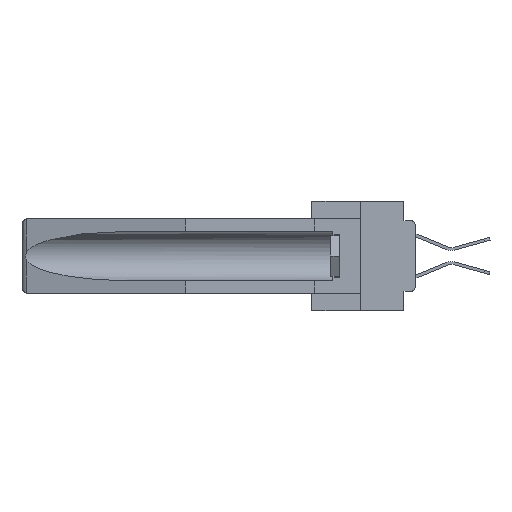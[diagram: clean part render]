
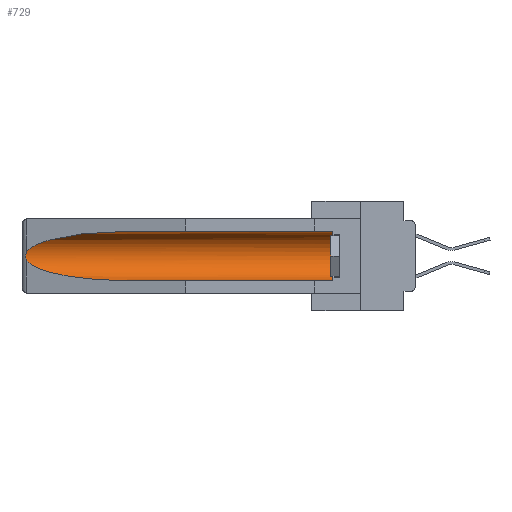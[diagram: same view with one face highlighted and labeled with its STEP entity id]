
A CAD part, left-side view. The second image highlights one B-rep face of the part: STEP entity #729.
In plain terms, the highlighted cylindrical face has radius 2.857 mm (diameter 5.715 mm), a partial arc.
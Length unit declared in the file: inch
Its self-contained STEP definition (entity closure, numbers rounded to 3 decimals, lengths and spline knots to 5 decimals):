
#336 = CARTESIAN_POINT ( 'NONE',  ( 0.155, -0.30754, -0.284 ) ) ;
#729 = ADVANCED_FACE ( 'NONE', ( #14350 ), #22308, .F. ) ;
#968 = CARTESIAN_POINT ( 'NONE',  ( 0.155, 1.07973, -0.284 ) ) ;
#1358 = ORIENTED_EDGE ( 'NONE', *, *, #25346, .T. ) ;
#1753 = EDGE_CURVE ( 'NONE', #28418, #22127, #26132, .T. ) ;
#1892 = DIRECTION ( 'NONE',  ( 0., 1., 0. ) ) ;
#1933 = CARTESIAN_POINT ( 'NONE',  ( 0.26654, 1.53092, -0.15636 ) ) ;
#2085 = CARTESIAN_POINT ( 'NONE',  ( 0.2675, 1.53308, -0.16763 ) ) ;
#2621 = CARTESIAN_POINT ( 'NONE',  ( 0.25451, 1.48313, -0.24835 ) ) ;
#4347 = CARTESIAN_POINT ( 'NONE',  ( 0.155, -0.30754, -0.1715 ) ) ;
#4593 = VECTOR ( 'NONE', #5719, 39.37008 ) ;
#5233 = CARTESIAN_POINT ( 'NONE',  ( 0.155, 1.07973, -0.284 ) ) ;
#5643 = CARTESIAN_POINT ( 'NONE',  ( 0.155, -0.30754, -0.059 ) ) ;
#5719 = DIRECTION ( 'NONE',  ( 0., 1., 0. ) ) ;
#6481 = ORIENTED_EDGE ( 'NONE', *, *, #31178, .T. ) ;
#7720 = EDGE_LOOP ( 'NONE', ( #1358, #6481, #26420, #23361, #24828, #29363 ) ) ;
#8289 = VERTEX_POINT ( 'NONE', #15054 ) ;
#8754 = LINE ( 'NONE', #5643, #9029 ) ;
#9025 = VERTEX_POINT ( 'NONE', #968 ) ;
#9029 = VECTOR ( 'NONE', #1892, 39.37008 ) ;
#10330 = CARTESIAN_POINT ( 'NONE',  ( 0.21114, 1.30732, -0.284 ) ) ;
#11923 = CARTESIAN_POINT ( 'NONE',  ( 0.26537, 1.52718, -0.19328 ) ) ;
#12438 = CARTESIAN_POINT ( 'NONE',  ( 0.155, 0.126, -0.1715 ) ) ;
#13761 = B_SPLINE_CURVE_WITH_KNOTS ( 'NONE', 3,
 ( #20060, #27481, #1933, #21863, #2085, #14536, #29668, #31794, #24609, #11923 ),
 .UNSPECIFIED., .F., .F.,
 ( 4, 2, 2, 2, 4 ),
 ( 0., 0.00029, 0.00058, 0.00087, 0.00117 ),
 .UNSPECIFIED. ) ;
#14350 = FACE_OUTER_BOUND ( 'NONE', #7720, .T. ) ;
#14536 = CARTESIAN_POINT ( 'NONE',  ( 0.2675, 1.53308, -0.17534 ) ) ;
#15054 = CARTESIAN_POINT ( 'NONE',  ( 0.26537, 1.52718, -0.14972 ) ) ;
#15680 = CARTESIAN_POINT ( 'NONE',  ( 0.26537, 1.52718, -0.19328 ) ) ;
#17288 = AXIS2_PLACEMENT_3D ( 'NONE', #12438, #24976, #30194 ) ;
#19222 = CARTESIAN_POINT ( 'NONE',  ( 0.155, 0.126, -0.284 ) ) ;
#19364 = CARTESIAN_POINT ( 'NONE',  ( 0.21114, 1.30732, -0.059 ) ) ;
#19534 = CARTESIAN_POINT ( 'NONE',  ( 0.26537, 1.52718, -0.14972 ) ) ;
#20060 = CARTESIAN_POINT ( 'NONE',  ( 0.26537, 1.52718, -0.14972 ) ) ;
#20889 = EDGE_CURVE ( 'NONE', #28418, #9025, #22883, .T. ) ;
#21863 = CARTESIAN_POINT ( 'NONE',  ( 0.2673, 1.5327, -0.16383 ) ) ;
#22005 = DIRECTION ( 'NONE',  ( 0., 0., 1. ) ) ;
#22127 = VERTEX_POINT ( 'NONE', #32031 ) ;
#22308 = CYLINDRICAL_SURFACE ( 'NONE', #28158, 0.1125 ) ;
#22883 = LINE ( 'NONE', #336, #4593 ) ;
#23361 = ORIENTED_EDGE ( 'NONE', *, *, #20889, .F. ) ;
#23392 = VERTEX_POINT ( 'NONE', #27031 ) ;
#24244 = CARTESIAN_POINT ( 'NONE',  ( 0.155, 1.07973, -0.059 ) ) ;
#24609 = CARTESIAN_POINT ( 'NONE',  ( 0.26597, 1.5296, -0.19026 ) ) ;
#24828 = ORIENTED_EDGE ( 'NONE', *, *, #1753, .T. ) ;
#24976 = DIRECTION ( 'NONE',  ( 0., -1., 0. ) ) ;
#25177 =( BOUNDED_CURVE ( )  B_SPLINE_CURVE ( 3, ( #24244, #19364, #27319, #19534 ),
 .UNSPECIFIED., .F., .T. ) 
 B_SPLINE_CURVE_WITH_KNOTS ( ( 4, 4 ),
 ( 4.71239, 6.08839 ),
 .UNSPECIFIED. ) 
 CURVE ( )  GEOMETRIC_REPRESENTATION_ITEM ( )  RATIONAL_B_SPLINE_CURVE ( ( 1., 0.848, 0.848, 1. ) ) 
 REPRESENTATION_ITEM ( '' )  );
#25346 = EDGE_CURVE ( 'NONE', #23392, #8289, #25177, .T. ) ;
#25470 = CARTESIAN_POINT ( 'NONE',  ( 0.26537, 1.52718, -0.19328 ) ) ;
#25883 = EDGE_CURVE ( 'NONE', #27621, #9025, #26440, .T. ) ;
#26132 = CIRCLE ( 'NONE', #17288, 0.1125 ) ;
#26420 = ORIENTED_EDGE ( 'NONE', *, *, #25883, .T. ) ;
#26440 =( BOUNDED_CURVE ( )  B_SPLINE_CURVE ( 3, ( #25470, #2621, #10330, #5233 ),
 .UNSPECIFIED., .F., .T. ) 
 B_SPLINE_CURVE_WITH_KNOTS ( ( 4, 4 ),
 ( 0.1948, 1.5708 ),
 .UNSPECIFIED. ) 
 CURVE ( )  GEOMETRIC_REPRESENTATION_ITEM ( )  RATIONAL_B_SPLINE_CURVE ( ( 1., 0.848, 0.848, 1. ) ) 
 REPRESENTATION_ITEM ( '' )  );
#27031 = CARTESIAN_POINT ( 'NONE',  ( 0.155, 1.07973, -0.059 ) ) ;
#27319 = CARTESIAN_POINT ( 'NONE',  ( 0.25451, 1.48313, -0.09465 ) ) ;
#27481 = CARTESIAN_POINT ( 'NONE',  ( 0.26597, 1.52961, -0.15275 ) ) ;
#27621 = VERTEX_POINT ( 'NONE', #15680 ) ;
#28158 = AXIS2_PLACEMENT_3D ( 'NONE', #4347, #29799, #22005 ) ;
#28341 = EDGE_CURVE ( 'NONE', #22127, #23392, #8754, .T. ) ;
#28418 = VERTEX_POINT ( 'NONE', #19222 ) ;
#29363 = ORIENTED_EDGE ( 'NONE', *, *, #28341, .T. ) ;
#29668 = CARTESIAN_POINT ( 'NONE',  ( 0.2673, 1.53269, -0.17917 ) ) ;
#29799 = DIRECTION ( 'NONE',  ( 0., 1., 0. ) ) ;
#30194 = DIRECTION ( 'NONE',  ( 0., 0., 1. ) ) ;
#31178 = EDGE_CURVE ( 'NONE', #8289, #27621, #13761, .T. ) ;
#31794 = CARTESIAN_POINT ( 'NONE',  ( 0.26655, 1.53094, -0.18657 ) ) ;
#32031 = CARTESIAN_POINT ( 'NONE',  ( 0.155, 0.126, -0.059 ) ) ;
